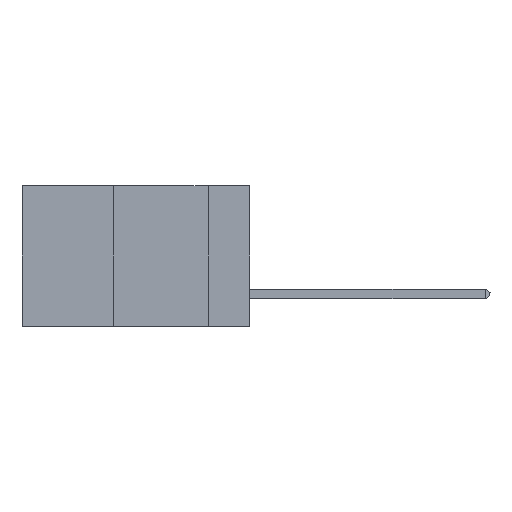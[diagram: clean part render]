
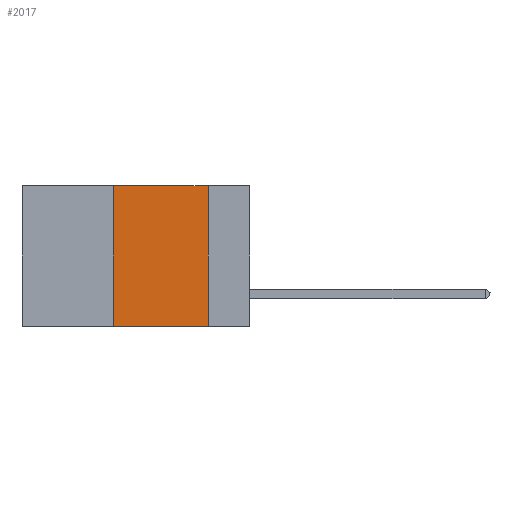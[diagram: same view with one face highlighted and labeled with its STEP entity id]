
A CAD part, left-side view. The second image highlights one B-rep face of the part: STEP entity #2017.
In plain terms, the highlighted planar face has unit normal (-1, 0, 0).
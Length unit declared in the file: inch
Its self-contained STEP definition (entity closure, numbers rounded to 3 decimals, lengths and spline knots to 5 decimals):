
#165 = EDGE_CURVE ( 'NONE', #1468, #10334, #5719, .T. ) ;
#227 = CARTESIAN_POINT ( 'NONE',  ( 0., 0.6, 0. ) ) ;
#480 = FACE_OUTER_BOUND ( 'NONE', #4533, .T. ) ;
#974 = DIRECTION ( 'NONE',  ( 0., -1., 0. ) ) ;
#1468 = VERTEX_POINT ( 'NONE', #8579 ) ;
#1625 = CARTESIAN_POINT ( 'NONE',  ( 0., 0.11, 0. ) ) ;
#1862 = DIRECTION ( 'NONE',  ( 1., 0., 0. ) ) ;
#2017 = ADVANCED_FACE ( 'NONE', ( #480 ), #9550, .F. ) ;
#2117 = VERTEX_POINT ( 'NONE', #1625 ) ;
#2510 = ORIENTED_EDGE ( 'NONE', *, *, #165, .T. ) ;
#3387 = ORIENTED_EDGE ( 'NONE', *, *, #14084, .F. ) ;
#3608 = CARTESIAN_POINT ( 'NONE',  ( 0., 0.11, 0. ) ) ;
#3995 = LINE ( 'NONE', #227, #4187 ) ;
#4187 = VECTOR ( 'NONE', #12417, 39.37008 ) ;
#4323 = DIRECTION ( 'NONE',  ( 0., 0., 1. ) ) ;
#4533 = EDGE_LOOP ( 'NONE', ( #3387, #7639, #8057, #2510 ) ) ;
#5719 = LINE ( 'NONE', #12496, #10602 ) ;
#6009 = VECTOR ( 'NONE', #13656, 39.37008 ) ;
#6026 = AXIS2_PLACEMENT_3D ( 'NONE', #8504, #1862, #9596 ) ;
#6114 = VECTOR ( 'NONE', #4323, 39.37008 ) ;
#6449 = EDGE_CURVE ( 'NONE', #10821, #2117, #3995, .T. ) ;
#6557 = CARTESIAN_POINT ( 'NONE',  ( 0., 0.36, 0. ) ) ;
#6761 = CARTESIAN_POINT ( 'NONE',  ( 0., 0.36, 0. ) ) ;
#6990 = CARTESIAN_POINT ( 'NONE',  ( 0., 0.11, -0.37 ) ) ;
#7431 = EDGE_CURVE ( 'NONE', #1468, #10821, #12216, .T. ) ;
#7639 = ORIENTED_EDGE ( 'NONE', *, *, #6449, .F. ) ;
#8057 = ORIENTED_EDGE ( 'NONE', *, *, #7431, .F. ) ;
#8504 = CARTESIAN_POINT ( 'NONE',  ( 0., 0.6, 0. ) ) ;
#8579 = CARTESIAN_POINT ( 'NONE',  ( 0., 0.36, -0.37 ) ) ;
#9550 = PLANE ( 'NONE',  #6026 ) ;
#9596 = DIRECTION ( 'NONE',  ( 0., 0., -1. ) ) ;
#10334 = VERTEX_POINT ( 'NONE', #6990 ) ;
#10372 = LINE ( 'NONE', #3608, #6009 ) ;
#10602 = VECTOR ( 'NONE', #974, 39.37008 ) ;
#10821 = VERTEX_POINT ( 'NONE', #6761 ) ;
#12216 = LINE ( 'NONE', #6557, #6114 ) ;
#12417 = DIRECTION ( 'NONE',  ( 0., -1., 0. ) ) ;
#12496 = CARTESIAN_POINT ( 'NONE',  ( 0., 0.6, -0.37 ) ) ;
#13656 = DIRECTION ( 'NONE',  ( 0., 0., -1. ) ) ;
#14084 = EDGE_CURVE ( 'NONE', #2117, #10334, #10372, .T. ) ;
